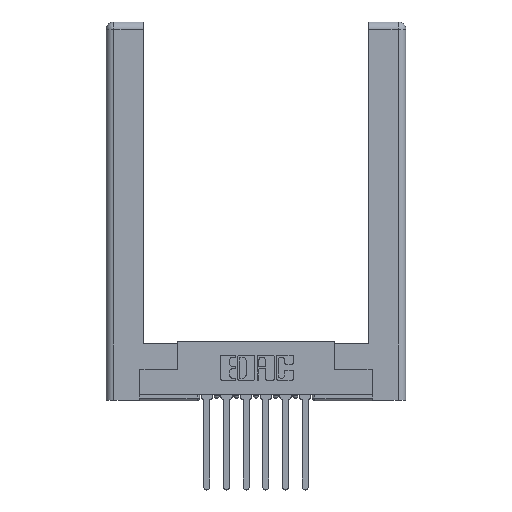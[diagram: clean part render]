
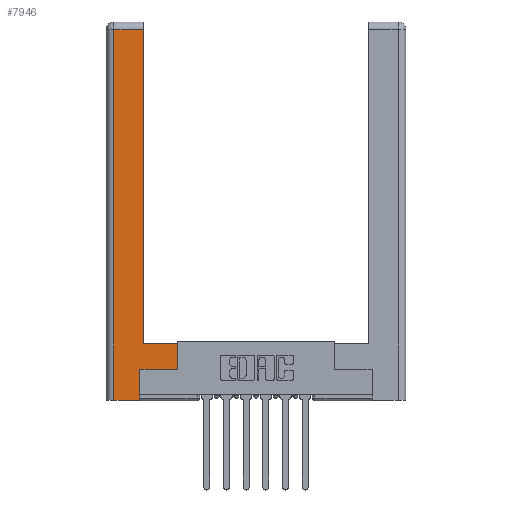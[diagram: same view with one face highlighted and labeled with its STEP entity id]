
A CAD part, top view. The second image highlights one B-rep face of the part: STEP entity #7946.
In plain terms, the highlighted planar face has unit normal (0, 0, 1).
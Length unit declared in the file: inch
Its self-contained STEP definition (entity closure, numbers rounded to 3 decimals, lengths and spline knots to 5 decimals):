
#361 = EDGE_CURVE ( 'NONE', #6972, #4947, #8579, .T. ) ;
#544 = CARTESIAN_POINT ( 'NONE',  ( 0.265, 0., 0. ) ) ;
#779 = VERTEX_POINT ( 'NONE', #4728 ) ;
#805 = CARTESIAN_POINT ( 'NONE',  ( 0.265, 0.245, 0. ) ) ;
#835 = CARTESIAN_POINT ( 'NONE',  ( 0.565, 0.45, 0. ) ) ;
#981 = ORIENTED_EDGE ( 'NONE', *, *, #11882, .T. ) ;
#1069 = DIRECTION ( 'NONE',  ( 0., 1., 0. ) ) ;
#1441 = VECTOR ( 'NONE', #10146, 39.37008 ) ;
#1503 = VERTEX_POINT ( 'NONE', #12190 ) ;
#1872 = DIRECTION ( 'NONE',  ( 0., 1., 0. ) ) ;
#1883 = ORIENTED_EDGE ( 'NONE', *, *, #361, .T. ) ;
#2010 = CARTESIAN_POINT ( 'NONE',  ( 0.565, 0.45, 0. ) ) ;
#2082 = LINE ( 'NONE', #4955, #10121 ) ;
#3289 = DIRECTION ( 'NONE',  ( -1., 0., 0. ) ) ;
#3530 = CARTESIAN_POINT ( 'NONE',  ( 0.295, 0.45, 0. ) ) ;
#3754 = DIRECTION ( 'NONE',  ( -1., 0., 0. ) ) ;
#3896 = EDGE_CURVE ( 'NONE', #12388, #1503, #9719, .T. ) ;
#4362 = ORIENTED_EDGE ( 'NONE', *, *, #6294, .T. ) ;
#4728 = CARTESIAN_POINT ( 'NONE',  ( 0.0615, 0., 0. ) ) ;
#4947 = VERTEX_POINT ( 'NONE', #5165 ) ;
#4955 = CARTESIAN_POINT ( 'NONE',  ( 0.0615, 0., 0. ) ) ;
#5165 = CARTESIAN_POINT ( 'NONE',  ( 0.295, 2.94, 0. ) ) ;
#5290 = EDGE_CURVE ( 'NONE', #8257, #779, #2082, .T. ) ;
#5468 = ORIENTED_EDGE ( 'NONE', *, *, #3896, .T. ) ;
#5670 = LINE ( 'NONE', #7608, #7021 ) ;
#5797 = VECTOR ( 'NONE', #1069, 39.37008 ) ;
#5973 = DIRECTION ( 'NONE',  ( 1., 0., 0. ) ) ;
#6215 = EDGE_CURVE ( 'NONE', #11408, #12388, #10655, .T. ) ;
#6294 = EDGE_CURVE ( 'NONE', #1503, #8768, #6781, .T. ) ;
#6640 = FACE_OUTER_BOUND ( 'NONE', #6684, .T. ) ;
#6684 = EDGE_LOOP ( 'NONE', ( #1883, #11729, #8845, #981, #6931, #5468, #4362, #11557 ) ) ;
#6781 = LINE ( 'NONE', #2010, #5797 ) ;
#6931 = ORIENTED_EDGE ( 'NONE', *, *, #6215, .T. ) ;
#6972 = VERTEX_POINT ( 'NONE', #10069 ) ;
#7021 = VECTOR ( 'NONE', #7485, 39.37008 ) ;
#7396 = VECTOR ( 'NONE', #11400, 39.37008 ) ;
#7416 = EDGE_CURVE ( 'NONE', #8768, #6972, #8230, .T. ) ;
#7485 = DIRECTION ( 'NONE',  ( -1., 0., 0. ) ) ;
#7608 = CARTESIAN_POINT ( 'NONE',  ( 0.0615, 2.94, 0. ) ) ;
#7708 = DIRECTION ( 'NONE',  ( 0., 0., -1. ) ) ;
#7946 = ADVANCED_FACE ( 'NONE', ( #6640 ), #8464, .F. ) ;
#8199 = LINE ( 'NONE', #544, #1441 ) ;
#8230 = LINE ( 'NONE', #3530, #9467 ) ;
#8252 = CARTESIAN_POINT ( 'NONE',  ( 0.0615, 2.94, 0. ) ) ;
#8257 = VERTEX_POINT ( 'NONE', #8252 ) ;
#8464 = PLANE ( 'NONE',  #8899 ) ;
#8579 = LINE ( 'NONE', #9697, #10214 ) ;
#8768 = VERTEX_POINT ( 'NONE', #835 ) ;
#8789 = CARTESIAN_POINT ( 'NONE',  ( 0.565, 0.245, 0. ) ) ;
#8845 = ORIENTED_EDGE ( 'NONE', *, *, #5290, .T. ) ;
#8899 = AXIS2_PLACEMENT_3D ( 'NONE', #10387, #7708, #3754 ) ;
#9131 = CARTESIAN_POINT ( 'NONE',  ( 0.265, 0.245, 0. ) ) ;
#9467 = VECTOR ( 'NONE', #3289, 39.37008 ) ;
#9697 = CARTESIAN_POINT ( 'NONE',  ( 0.295, 3., 0. ) ) ;
#9719 = LINE ( 'NONE', #8789, #10497 ) ;
#9778 = DIRECTION ( 'NONE',  ( 0., -1., 0. ) ) ;
#10069 = CARTESIAN_POINT ( 'NONE',  ( 0.295, 0.45, 0. ) ) ;
#10121 = VECTOR ( 'NONE', #9778, 39.37008 ) ;
#10146 = DIRECTION ( 'NONE',  ( 1., 0., 0. ) ) ;
#10214 = VECTOR ( 'NONE', #1872, 39.37008 ) ;
#10241 = EDGE_CURVE ( 'NONE', #4947, #8257, #5670, .T. ) ;
#10387 = CARTESIAN_POINT ( 'NONE',  ( 0., 0., 0. ) ) ;
#10497 = VECTOR ( 'NONE', #5973, 39.37008 ) ;
#10655 = LINE ( 'NONE', #805, #7396 ) ;
#11400 = DIRECTION ( 'NONE',  ( 0., 1., 0. ) ) ;
#11408 = VERTEX_POINT ( 'NONE', #11848 ) ;
#11557 = ORIENTED_EDGE ( 'NONE', *, *, #7416, .T. ) ;
#11729 = ORIENTED_EDGE ( 'NONE', *, *, #10241, .T. ) ;
#11848 = CARTESIAN_POINT ( 'NONE',  ( 0.265, 0., 0. ) ) ;
#11882 = EDGE_CURVE ( 'NONE', #779, #11408, #8199, .T. ) ;
#12190 = CARTESIAN_POINT ( 'NONE',  ( 0.565, 0.245, 0. ) ) ;
#12388 = VERTEX_POINT ( 'NONE', #9131 ) ;
